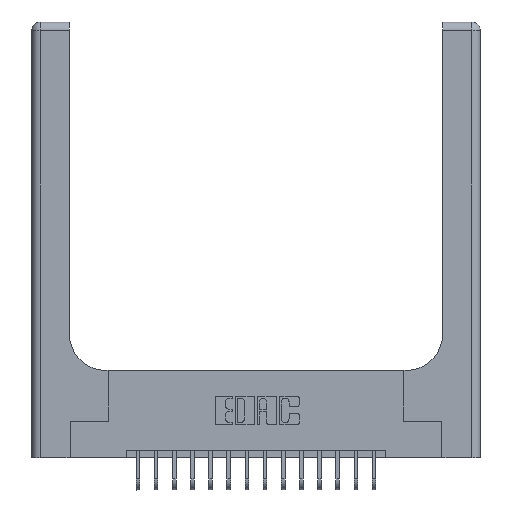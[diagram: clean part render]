
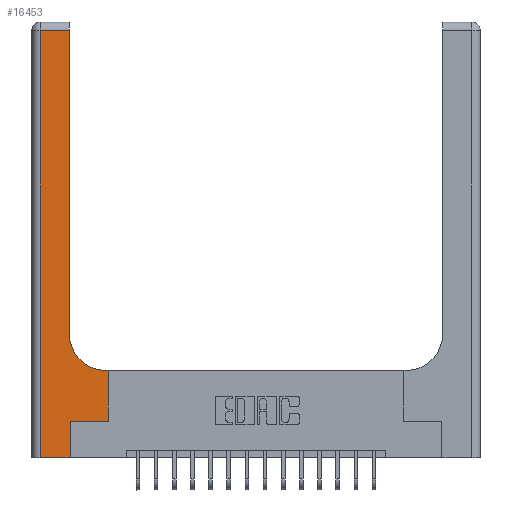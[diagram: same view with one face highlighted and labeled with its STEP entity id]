
A CAD part, top view. The second image highlights one B-rep face of the part: STEP entity #16453.
In plain terms, the highlighted planar face has unit normal (0, 0, 1).
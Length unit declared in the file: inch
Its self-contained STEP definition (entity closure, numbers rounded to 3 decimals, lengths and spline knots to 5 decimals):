
#88 = CARTESIAN_POINT ( 'NONE',  ( 0.265, 0., 0.37 ) ) ;
#219 = DIRECTION ( 'NONE',  ( -1., 0., 0. ) ) ;
#310 = VECTOR ( 'NONE', #12914, 39.37008 ) ;
#312 = EDGE_CURVE ( 'NONE', #6245, #9216, #19238, .T. ) ;
#420 = LINE ( 'NONE', #9883, #9908 ) ;
#524 = VERTEX_POINT ( 'NONE', #7697 ) ;
#687 = VERTEX_POINT ( 'NONE', #88 ) ;
#1181 = CARTESIAN_POINT ( 'NONE',  ( 0.265, 0.25, 0.37 ) ) ;
#1432 = ORIENTED_EDGE ( 'NONE', *, *, #7565, .T. ) ;
#2686 = CARTESIAN_POINT ( 'NONE',  ( 0.528, 0.25, 0.37 ) ) ;
#3530 = CARTESIAN_POINT ( 'NONE',  ( 0.528, 0.6, 0.37 ) ) ;
#3591 = EDGE_CURVE ( 'NONE', #17651, #20120, #20304, .T. ) ;
#3718 = EDGE_CURVE ( 'NONE', #9216, #524, #5073, .T. ) ;
#4469 = VECTOR ( 'NONE', #13590, 39.37008 ) ;
#4617 = DIRECTION ( 'NONE',  ( 1., 0., 0. ) ) ;
#5073 = LINE ( 'NONE', #8075, #310 ) ;
#5132 = CARTESIAN_POINT ( 'NONE',  ( 0.26, 3., 0.37 ) ) ;
#5241 = DIRECTION ( 'NONE',  ( 0., -1., 0. ) ) ;
#5816 = CARTESIAN_POINT ( 'NONE',  ( 0.06, 0., 0.37 ) ) ;
#5819 = DIRECTION ( 'NONE',  ( -1., 0., 0. ) ) ;
#5887 = AXIS2_PLACEMENT_3D ( 'NONE', #6695, #16641, #18086 ) ;
#6037 = VECTOR ( 'NONE', #4617, 39.37008 ) ;
#6245 = VERTEX_POINT ( 'NONE', #9757 ) ;
#6537 = EDGE_CURVE ( 'NONE', #18715, #10861, #12209, .T. ) ;
#6695 = CARTESIAN_POINT ( 'NONE',  ( 0.51, 0.85, 0.37 ) ) ;
#6795 = DIRECTION ( 'NONE',  ( 0., 0., -1. ) ) ;
#6986 = CARTESIAN_POINT ( 'NONE',  ( 0.265, 0., 0.37 ) ) ;
#7187 = VECTOR ( 'NONE', #9007, 39.37008 ) ;
#7565 = EDGE_CURVE ( 'NONE', #10861, #6245, #7875, .T. ) ;
#7697 = CARTESIAN_POINT ( 'NONE',  ( 0.06, 2.94, 0.37 ) ) ;
#7724 = ORIENTED_EDGE ( 'NONE', *, *, #3591, .T. ) ;
#7875 = CIRCLE ( 'NONE', #5887, 0.25 ) ;
#7989 = ORIENTED_EDGE ( 'NONE', *, *, #18859, .T. ) ;
#8075 = CARTESIAN_POINT ( 'NONE',  ( 0., 2.94, 0.37 ) ) ;
#8145 = PLANE ( 'NONE',  #19201 ) ;
#8244 = FACE_OUTER_BOUND ( 'NONE', #14223, .T. ) ;
#8344 = CARTESIAN_POINT ( 'NONE',  ( 0., 3., 0.37 ) ) ;
#9007 = DIRECTION ( 'NONE',  ( 1., 0., 0. ) ) ;
#9078 = CARTESIAN_POINT ( 'NONE',  ( 0.528, 0.25, 0.37 ) ) ;
#9119 = LINE ( 'NONE', #6986, #20204 ) ;
#9216 = VERTEX_POINT ( 'NONE', #12451 ) ;
#9532 = VECTOR ( 'NONE', #5819, 39.37008 ) ;
#9757 = CARTESIAN_POINT ( 'NONE',  ( 0.26, 0.85, 0.37 ) ) ;
#9883 = CARTESIAN_POINT ( 'NONE',  ( 0.06, 3., 0.37 ) ) ;
#9908 = VECTOR ( 'NONE', #5241, 39.37008 ) ;
#10148 = EDGE_CURVE ( 'NONE', #524, #14120, #420, .T. ) ;
#10491 = ORIENTED_EDGE ( 'NONE', *, *, #3718, .T. ) ;
#10861 = VERTEX_POINT ( 'NONE', #12706 ) ;
#12209 = LINE ( 'NONE', #15194, #9532 ) ;
#12292 = ORIENTED_EDGE ( 'NONE', *, *, #6537, .T. ) ;
#12294 = VECTOR ( 'NONE', #14303, 39.37008 ) ;
#12451 = CARTESIAN_POINT ( 'NONE',  ( 0.26, 2.94, 0.37 ) ) ;
#12706 = CARTESIAN_POINT ( 'NONE',  ( 0.51, 0.6, 0.37 ) ) ;
#12914 = DIRECTION ( 'NONE',  ( -1., 0., 0. ) ) ;
#13522 = ORIENTED_EDGE ( 'NONE', *, *, #312, .T. ) ;
#13590 = DIRECTION ( 'NONE',  ( 0., 1., 0. ) ) ;
#13799 = LINE ( 'NONE', #2686, #4469 ) ;
#14120 = VERTEX_POINT ( 'NONE', #5816 ) ;
#14223 = EDGE_LOOP ( 'NONE', ( #13522, #10491, #20176, #18821, #16501, #7724, #7989, #12292, #1432 ) ) ;
#14303 = DIRECTION ( 'NONE',  ( 0., 1., 0. ) ) ;
#15194 = CARTESIAN_POINT ( 'NONE',  ( 0.26, 0.6, 0.37 ) ) ;
#15502 = DIRECTION ( 'NONE',  ( 0., 1., 0. ) ) ;
#15639 = LINE ( 'NONE', #18719, #6037 ) ;
#16453 = ADVANCED_FACE ( 'NONE', ( #8244 ), #8145, .F. ) ;
#16501 = ORIENTED_EDGE ( 'NONE', *, *, #17913, .T. ) ;
#16641 = DIRECTION ( 'NONE',  ( 0., 0., -1. ) ) ;
#16779 = EDGE_CURVE ( 'NONE', #14120, #687, #15639, .T. ) ;
#17651 = VERTEX_POINT ( 'NONE', #20157 ) ;
#17913 = EDGE_CURVE ( 'NONE', #687, #17651, #9119, .T. ) ;
#18086 = DIRECTION ( 'NONE',  ( 1., 0., 0. ) ) ;
#18715 = VERTEX_POINT ( 'NONE', #3530 ) ;
#18719 = CARTESIAN_POINT ( 'NONE',  ( 0., 0., 0.37 ) ) ;
#18821 = ORIENTED_EDGE ( 'NONE', *, *, #16779, .T. ) ;
#18859 = EDGE_CURVE ( 'NONE', #20120, #18715, #13799, .T. ) ;
#19201 = AXIS2_PLACEMENT_3D ( 'NONE', #8344, #6795, #219 ) ;
#19238 = LINE ( 'NONE', #5132, #12294 ) ;
#20120 = VERTEX_POINT ( 'NONE', #9078 ) ;
#20157 = CARTESIAN_POINT ( 'NONE',  ( 0.265, 0.25, 0.37 ) ) ;
#20176 = ORIENTED_EDGE ( 'NONE', *, *, #10148, .T. ) ;
#20204 = VECTOR ( 'NONE', #15502, 39.37008 ) ;
#20304 = LINE ( 'NONE', #1181, #7187 ) ;
